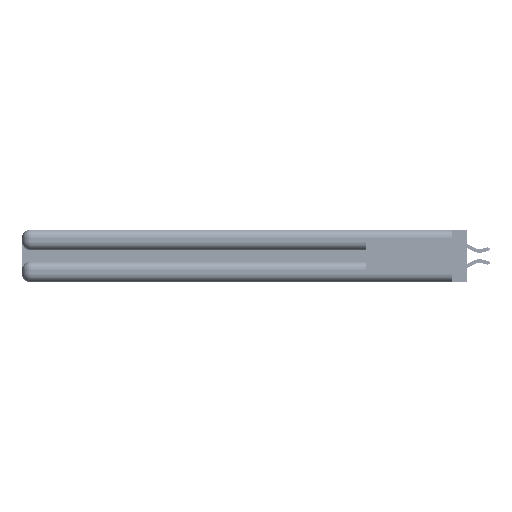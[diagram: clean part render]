
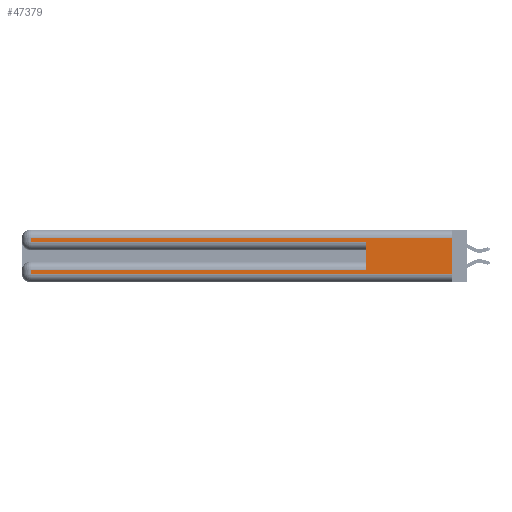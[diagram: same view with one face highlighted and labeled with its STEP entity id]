
A CAD part, left-side view. The second image highlights one B-rep face of the part: STEP entity #47379.
In plain terms, the highlighted planar face has unit normal (-1, 0, 0).
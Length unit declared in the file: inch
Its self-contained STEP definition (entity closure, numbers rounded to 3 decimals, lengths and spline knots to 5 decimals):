
#926 = CARTESIAN_POINT ( 'NONE',  ( 0., 2.94, 0.37 ) ) ;
#1727 = CARTESIAN_POINT ( 'NONE',  ( 0., 0., 0.31 ) ) ;
#3815 = VERTEX_POINT ( 'NONE', #17528 ) ;
#3951 = LINE ( 'NONE', #42936, #24662 ) ;
#4640 = VECTOR ( 'NONE', #15211, 39.37008 ) ;
#5755 = CARTESIAN_POINT ( 'NONE',  ( 0., 2.94, 0.285 ) ) ;
#6122 = VECTOR ( 'NONE', #11554, 39.37008 ) ;
#6710 = FACE_OUTER_BOUND ( 'NONE', #17973, .T. ) ;
#7827 = CARTESIAN_POINT ( 'NONE',  ( 0., 0., 0.37 ) ) ;
#8022 = CARTESIAN_POINT ( 'NONE',  ( 0., 0., 0.06 ) ) ;
#8352 = ORIENTED_EDGE ( 'NONE', *, *, #50744, .T. ) ;
#9564 = VECTOR ( 'NONE', #30688, 39.37008 ) ;
#9720 = CARTESIAN_POINT ( 'NONE',  ( 0., 2.94, 0.085 ) ) ;
#11554 = DIRECTION ( 'NONE',  ( 0., 1., 0. ) ) ;
#12030 = CARTESIAN_POINT ( 'NONE',  ( 0., 0.6, 0.085 ) ) ;
#12490 = DIRECTION ( 'NONE',  ( 0., 0., 1. ) ) ;
#13284 = CARTESIAN_POINT ( 'NONE',  ( 0., 2.94, 0.06 ) ) ;
#15211 = DIRECTION ( 'NONE',  ( 0., 0., -1. ) ) ;
#15706 = LINE ( 'NONE', #926, #24089 ) ;
#16166 = PLANE ( 'NONE',  #48937 ) ;
#17528 = CARTESIAN_POINT ( 'NONE',  ( 0., 2.94, 0.31 ) ) ;
#17614 = VERTEX_POINT ( 'NONE', #13284 ) ;
#17637 = DIRECTION ( 'NONE',  ( 0., 0., -1. ) ) ;
#17973 = EDGE_LOOP ( 'NONE', ( #51083, #30212, #32058, #52807, #22341, #41655, #53063, #8352 ) ) ;
#19305 = LINE ( 'NONE', #8022, #50839 ) ;
#20321 = DIRECTION ( 'NONE',  ( 0., 0., -1. ) ) ;
#22341 = ORIENTED_EDGE ( 'NONE', *, *, #43543, .F. ) ;
#23408 = EDGE_CURVE ( 'NONE', #3815, #41765, #15706, .T. ) ;
#23587 = CARTESIAN_POINT ( 'NONE',  ( 0., 0.6, 0.145 ) ) ;
#23664 = CARTESIAN_POINT ( 'NONE',  ( 0., 0., 0.31 ) ) ;
#23898 = LINE ( 'NONE', #33165, #44525 ) ;
#24089 = VECTOR ( 'NONE', #17637, 39.37008 ) ;
#24547 = CARTESIAN_POINT ( 'NONE',  ( 0., 0., 0.06 ) ) ;
#24645 = DIRECTION ( 'NONE',  ( 0., -1., 0. ) ) ;
#24662 = VECTOR ( 'NONE', #30700, 39.37008 ) ;
#25170 = VERTEX_POINT ( 'NONE', #12030 ) ;
#25919 = EDGE_CURVE ( 'NONE', #41765, #44698, #23898, .T. ) ;
#27900 = VECTOR ( 'NONE', #12490, 39.37008 ) ;
#29705 = EDGE_CURVE ( 'NONE', #51871, #46174, #48533, .T. ) ;
#30212 = ORIENTED_EDGE ( 'NONE', *, *, #52232, .T. ) ;
#30247 = LINE ( 'NONE', #1727, #9564 ) ;
#30688 = DIRECTION ( 'NONE',  ( 0., 1., 0. ) ) ;
#30700 = DIRECTION ( 'NONE',  ( 0., 0., -1. ) ) ;
#32058 = ORIENTED_EDGE ( 'NONE', *, *, #23408, .T. ) ;
#33165 = CARTESIAN_POINT ( 'NONE',  ( 0., 0., 0.285 ) ) ;
#37219 = EDGE_CURVE ( 'NONE', #48340, #17614, #3951, .T. ) ;
#40522 = CARTESIAN_POINT ( 'NONE',  ( 0., 0.6, 0.285 ) ) ;
#41442 = LINE ( 'NONE', #23587, #27900 ) ;
#41655 = ORIENTED_EDGE ( 'NONE', *, *, #46048, .T. ) ;
#41765 = VERTEX_POINT ( 'NONE', #5755 ) ;
#42936 = CARTESIAN_POINT ( 'NONE',  ( 0., 2.94, 0.37 ) ) ;
#43543 = EDGE_CURVE ( 'NONE', #25170, #44698, #41442, .T. ) ;
#44525 = VECTOR ( 'NONE', #49462, 39.37008 ) ;
#44698 = VERTEX_POINT ( 'NONE', #40522 ) ;
#44993 = DIRECTION ( 'NONE',  ( 1., 0., 0. ) ) ;
#46048 = EDGE_CURVE ( 'NONE', #25170, #48340, #51289, .T. ) ;
#46174 = VERTEX_POINT ( 'NONE', #24547 ) ;
#47379 = ADVANCED_FACE ( 'NONE', ( #6710 ), #16166, .F. ) ;
#48340 = VERTEX_POINT ( 'NONE', #9720 ) ;
#48533 = LINE ( 'NONE', #52099, #4640 ) ;
#48937 = AXIS2_PLACEMENT_3D ( 'NONE', #7827, #44993, #20321 ) ;
#49462 = DIRECTION ( 'NONE',  ( 0., -1., 0. ) ) ;
#50744 = EDGE_CURVE ( 'NONE', #17614, #46174, #19305, .T. ) ;
#50839 = VECTOR ( 'NONE', #24645, 39.37008 ) ;
#51083 = ORIENTED_EDGE ( 'NONE', *, *, #29705, .F. ) ;
#51289 = LINE ( 'NONE', #52604, #6122 ) ;
#51871 = VERTEX_POINT ( 'NONE', #23664 ) ;
#52099 = CARTESIAN_POINT ( 'NONE',  ( 0., 0., 0.37 ) ) ;
#52232 = EDGE_CURVE ( 'NONE', #51871, #3815, #30247, .T. ) ;
#52604 = CARTESIAN_POINT ( 'NONE',  ( 0., 0., 0.085 ) ) ;
#52807 = ORIENTED_EDGE ( 'NONE', *, *, #25919, .T. ) ;
#53063 = ORIENTED_EDGE ( 'NONE', *, *, #37219, .T. ) ;
